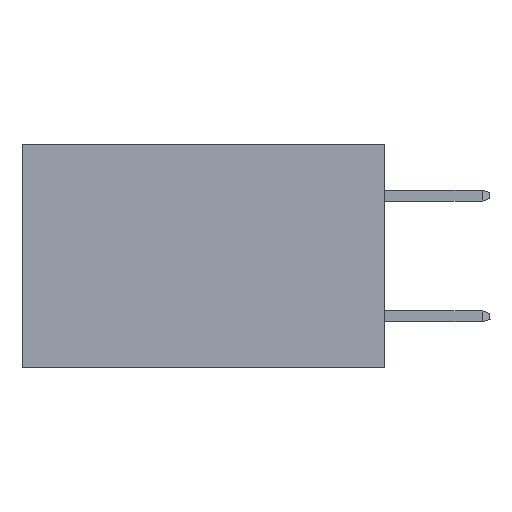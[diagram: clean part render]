
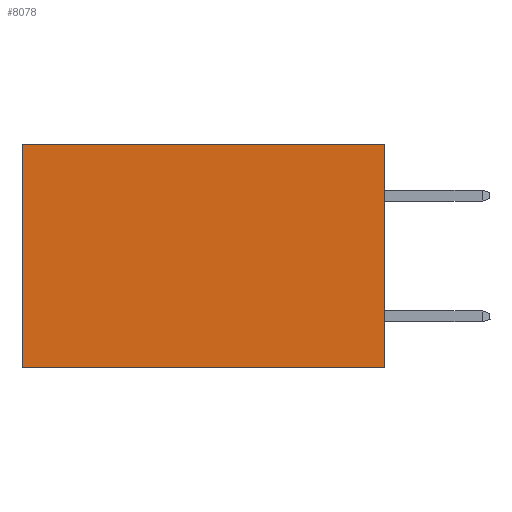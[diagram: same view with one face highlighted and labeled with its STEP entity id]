
A CAD part, left-side view. The second image highlights one B-rep face of the part: STEP entity #8078.
In plain terms, the highlighted planar face has unit normal (-1, 0, 0).
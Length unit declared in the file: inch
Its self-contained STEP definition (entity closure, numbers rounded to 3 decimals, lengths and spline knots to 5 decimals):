
#407 = VERTEX_POINT ( 'NONE', #8610 ) ;
#538 = CARTESIAN_POINT ( 'NONE',  ( 0.2615, 0.6, -0.37 ) ) ;
#3601 = EDGE_CURVE ( 'NONE', #407, #11240, #14858, .T. ) ;
#3972 = VERTEX_POINT ( 'NONE', #10629 ) ;
#4766 = ORIENTED_EDGE ( 'NONE', *, *, #16037, .T. ) ;
#5366 = VERTEX_POINT ( 'NONE', #8053 ) ;
#5917 = VECTOR ( 'NONE', #11239, 39.37008 ) ;
#6091 = EDGE_CURVE ( 'NONE', #5366, #407, #19518, .T. ) ;
#6101 = VECTOR ( 'NONE', #14702, 39.37008 ) ;
#6169 = VECTOR ( 'NONE', #19041, 39.37008 ) ;
#6276 = PLANE ( 'NONE',  #19885 ) ;
#6666 = LINE ( 'NONE', #538, #14830 ) ;
#7392 = DIRECTION ( 'NONE',  ( 0., 0., -1. ) ) ;
#7816 = FACE_OUTER_BOUND ( 'NONE', #11318, .T. ) ;
#8053 = CARTESIAN_POINT ( 'NONE',  ( 0.2615, 0., 0. ) ) ;
#8078 = ADVANCED_FACE ( 'NONE', ( #7816 ), #6276, .F. ) ;
#8321 = CARTESIAN_POINT ( 'NONE',  ( 0.2615, 0.6, -0.37 ) ) ;
#8610 = CARTESIAN_POINT ( 'NONE',  ( 0.2615, 0., -0.37 ) ) ;
#9247 = LINE ( 'NONE', #19285, #5917 ) ;
#9560 = CARTESIAN_POINT ( 'NONE',  ( 0.2615, 0., -0.37 ) ) ;
#10629 = CARTESIAN_POINT ( 'NONE',  ( 0.2615, 0.6, 0. ) ) ;
#11180 = DIRECTION ( 'NONE',  ( 0., 0., -1. ) ) ;
#11239 = DIRECTION ( 'NONE',  ( 0., 1., 0. ) ) ;
#11240 = VERTEX_POINT ( 'NONE', #8321 ) ;
#11318 = EDGE_LOOP ( 'NONE', ( #16923, #15219, #17347, #4766 ) ) ;
#11478 = EDGE_CURVE ( 'NONE', #3972, #11240, #6666, .T. ) ;
#14702 = DIRECTION ( 'NONE',  ( 0., 0., -1. ) ) ;
#14830 = VECTOR ( 'NONE', #7392, 39.37008 ) ;
#14858 = LINE ( 'NONE', #19104, #6169 ) ;
#15219 = ORIENTED_EDGE ( 'NONE', *, *, #3601, .F. ) ;
#16037 = EDGE_CURVE ( 'NONE', #5366, #3972, #9247, .T. ) ;
#16923 = ORIENTED_EDGE ( 'NONE', *, *, #11478, .T. ) ;
#17347 = ORIENTED_EDGE ( 'NONE', *, *, #6091, .F. ) ;
#19041 = DIRECTION ( 'NONE',  ( 0., 1., 0. ) ) ;
#19104 = CARTESIAN_POINT ( 'NONE',  ( 0.2615, 0., -0.37 ) ) ;
#19285 = CARTESIAN_POINT ( 'NONE',  ( 0.2615, 0., 0. ) ) ;
#19518 = LINE ( 'NONE', #21026, #6101 ) ;
#19885 = AXIS2_PLACEMENT_3D ( 'NONE', #9560, #20815, #11180 ) ;
#20815 = DIRECTION ( 'NONE',  ( 1., 0., 0. ) ) ;
#21026 = CARTESIAN_POINT ( 'NONE',  ( 0.2615, 0., -0.37 ) ) ;
